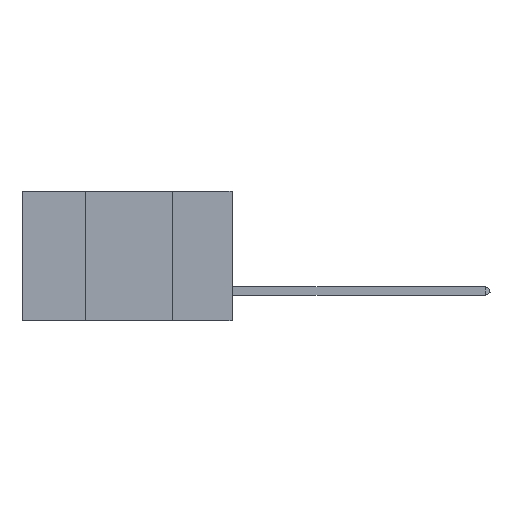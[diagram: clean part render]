
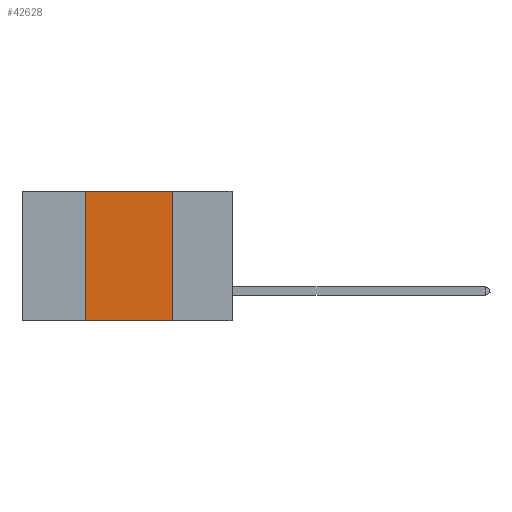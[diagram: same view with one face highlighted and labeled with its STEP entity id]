
A CAD part, left-side view. The second image highlights one B-rep face of the part: STEP entity #42628.
In plain terms, the highlighted planar face has unit normal (-1, 0, 0).
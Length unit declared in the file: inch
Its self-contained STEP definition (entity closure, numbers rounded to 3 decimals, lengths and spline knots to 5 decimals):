
#726 = CARTESIAN_POINT ( 'NONE',  ( 0., 0.17, -0.37 ) ) ;
#2457 = ORIENTED_EDGE ( 'NONE', *, *, #42720, .T. ) ;
#2831 = LINE ( 'NONE', #17974, #31140 ) ;
#3132 = PLANE ( 'NONE',  #37892 ) ;
#7002 = DIRECTION ( 'NONE',  ( 0., -1., 0. ) ) ;
#9653 = VECTOR ( 'NONE', #46596, 39.37008 ) ;
#11427 = CARTESIAN_POINT ( 'NONE',  ( 0., 0.42, 0. ) ) ;
#15490 = EDGE_CURVE ( 'NONE', #25893, #30743, #24042, .T. ) ;
#16885 = CARTESIAN_POINT ( 'NONE',  ( 0., 0.17, 0. ) ) ;
#17974 = CARTESIAN_POINT ( 'NONE',  ( 0., 0.6, -0.37 ) ) ;
#18842 = CARTESIAN_POINT ( 'NONE',  ( 0., 0.42, -0.37 ) ) ;
#20640 = CARTESIAN_POINT ( 'NONE',  ( 0., 0.17, 0. ) ) ;
#20804 = CARTESIAN_POINT ( 'NONE',  ( 0., 0.6, 0. ) ) ;
#21990 = VERTEX_POINT ( 'NONE', #18842 ) ;
#22471 = EDGE_CURVE ( 'NONE', #21990, #25893, #33981, .T. ) ;
#24042 = LINE ( 'NONE', #20804, #25779 ) ;
#24090 = FACE_OUTER_BOUND ( 'NONE', #27719, .T. ) ;
#25779 = VECTOR ( 'NONE', #43108, 39.37008 ) ;
#25893 = VERTEX_POINT ( 'NONE', #11427 ) ;
#26182 = LINE ( 'NONE', #20640, #34322 ) ;
#26500 = VERTEX_POINT ( 'NONE', #726 ) ;
#27719 = EDGE_LOOP ( 'NONE', ( #47269, #36990, #47483, #2457 ) ) ;
#30743 = VERTEX_POINT ( 'NONE', #16885 ) ;
#31140 = VECTOR ( 'NONE', #7002, 39.37008 ) ;
#31942 = CARTESIAN_POINT ( 'NONE',  ( 0., 0.42, 0. ) ) ;
#32303 = DIRECTION ( 'NONE',  ( 0., 0., -1. ) ) ;
#33981 = LINE ( 'NONE', #31942, #9653 ) ;
#34322 = VECTOR ( 'NONE', #32303, 39.37008 ) ;
#36440 = CARTESIAN_POINT ( 'NONE',  ( 0., 0.6, 0. ) ) ;
#36990 = ORIENTED_EDGE ( 'NONE', *, *, #15490, .F. ) ;
#37892 = AXIS2_PLACEMENT_3D ( 'NONE', #36440, #40127, #43032 ) ;
#40127 = DIRECTION ( 'NONE',  ( 1., 0., 0. ) ) ;
#42628 = ADVANCED_FACE ( 'NONE', ( #24090 ), #3132, .F. ) ;
#42720 = EDGE_CURVE ( 'NONE', #21990, #26500, #2831, .T. ) ;
#43032 = DIRECTION ( 'NONE',  ( 0., 0., -1. ) ) ;
#43108 = DIRECTION ( 'NONE',  ( 0., -1., 0. ) ) ;
#45162 = EDGE_CURVE ( 'NONE', #30743, #26500, #26182, .T. ) ;
#46596 = DIRECTION ( 'NONE',  ( 0., 0., 1. ) ) ;
#47269 = ORIENTED_EDGE ( 'NONE', *, *, #45162, .F. ) ;
#47483 = ORIENTED_EDGE ( 'NONE', *, *, #22471, .F. ) ;
